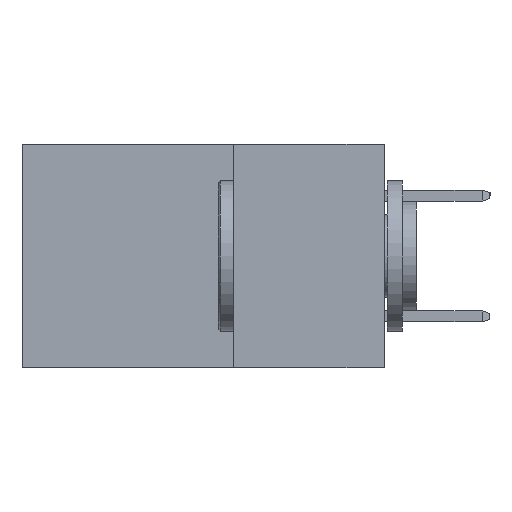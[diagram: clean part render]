
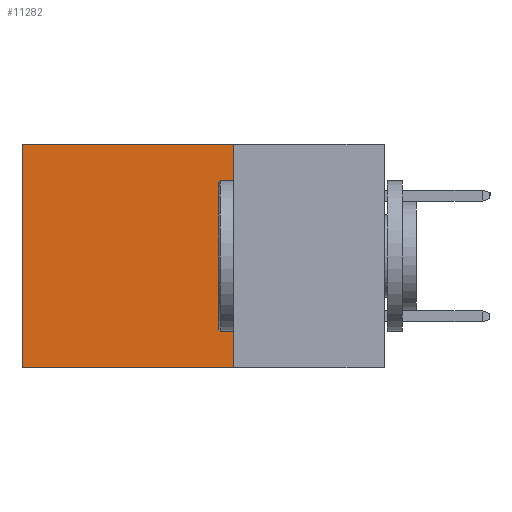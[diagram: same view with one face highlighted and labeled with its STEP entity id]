
A CAD part, left-side view. The second image highlights one B-rep face of the part: STEP entity #11282.
In plain terms, the highlighted planar face has unit normal (-1, 0, 0).
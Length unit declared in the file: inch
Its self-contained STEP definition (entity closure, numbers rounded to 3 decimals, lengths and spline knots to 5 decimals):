
#541 = CARTESIAN_POINT ( 'NONE',  ( 0.2615, 0.25, -0.37 ) ) ;
#830 = DIRECTION ( 'NONE',  ( 0., 0., -1. ) ) ;
#984 = DIRECTION ( 'NONE',  ( 0., 0., -1. ) ) ;
#1981 = DIRECTION ( 'NONE',  ( 0., 1., 0. ) ) ;
#2071 = LINE ( 'NONE', #20341, #11199 ) ;
#2306 = AXIS2_PLACEMENT_3D ( 'NONE', #16610, #19601, #8170 ) ;
#3080 = ORIENTED_EDGE ( 'NONE', *, *, #11423, .T. ) ;
#3083 = CARTESIAN_POINT ( 'NONE',  ( 0.2615, 0.6, -0.37 ) ) ;
#3879 = DIRECTION ( 'NONE',  ( 0., 1., 0. ) ) ;
#4359 = EDGE_CURVE ( 'NONE', #17505, #17243, #13787, .T. ) ;
#6029 = VERTEX_POINT ( 'NONE', #541 ) ;
#6578 = CARTESIAN_POINT ( 'NONE',  ( 0.2615, 0.25, 0. ) ) ;
#6679 = FACE_OUTER_BOUND ( 'NONE', #7147, .T. ) ;
#6870 = EDGE_CURVE ( 'NONE', #6029, #17243, #9985, .T. ) ;
#6915 = VERTEX_POINT ( 'NONE', #6578 ) ;
#7147 = EDGE_LOOP ( 'NONE', ( #13344, #19885, #16019, #3080 ) ) ;
#7865 = EDGE_CURVE ( 'NONE', #6915, #6029, #15362, .T. ) ;
#8170 = DIRECTION ( 'NONE',  ( 0., 0., -1. ) ) ;
#8375 = VECTOR ( 'NONE', #1981, 39.37008 ) ;
#9985 = LINE ( 'NONE', #15023, #8375 ) ;
#10042 = VECTOR ( 'NONE', #830, 39.37008 ) ;
#10105 = VECTOR ( 'NONE', #984, 39.37008 ) ;
#11199 = VECTOR ( 'NONE', #3879, 39.37008 ) ;
#11282 = ADVANCED_FACE ( 'NONE', ( #6679 ), #15013, .F. ) ;
#11423 = EDGE_CURVE ( 'NONE', #6915, #17505, #2071, .T. ) ;
#13344 = ORIENTED_EDGE ( 'NONE', *, *, #4359, .T. ) ;
#13787 = LINE ( 'NONE', #17326, #10105 ) ;
#13959 = CARTESIAN_POINT ( 'NONE',  ( 0.2615, 0.6, 0. ) ) ;
#15013 = PLANE ( 'NONE',  #2306 ) ;
#15023 = CARTESIAN_POINT ( 'NONE',  ( 0.2615, 0.25, -0.37 ) ) ;
#15362 = LINE ( 'NONE', #17163, #10042 ) ;
#16019 = ORIENTED_EDGE ( 'NONE', *, *, #7865, .F. ) ;
#16610 = CARTESIAN_POINT ( 'NONE',  ( 0.2615, 0.25, -0.37 ) ) ;
#17163 = CARTESIAN_POINT ( 'NONE',  ( 0.2615, 0.25, -0.37 ) ) ;
#17243 = VERTEX_POINT ( 'NONE', #3083 ) ;
#17326 = CARTESIAN_POINT ( 'NONE',  ( 0.2615, 0.6, -0.37 ) ) ;
#17505 = VERTEX_POINT ( 'NONE', #13959 ) ;
#19601 = DIRECTION ( 'NONE',  ( 1., 0., 0. ) ) ;
#19885 = ORIENTED_EDGE ( 'NONE', *, *, #6870, .F. ) ;
#20341 = CARTESIAN_POINT ( 'NONE',  ( 0.2615, 0.25, 0. ) ) ;
